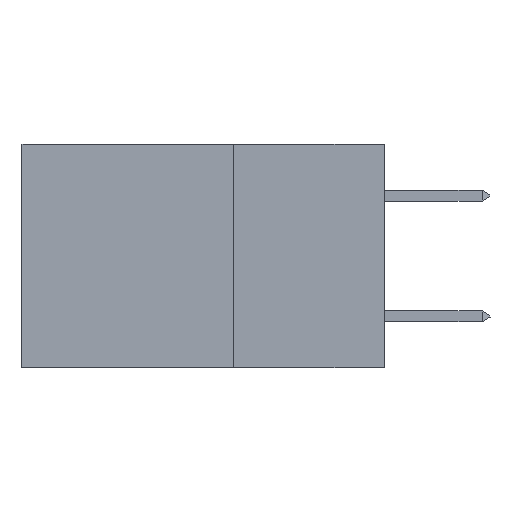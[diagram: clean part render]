
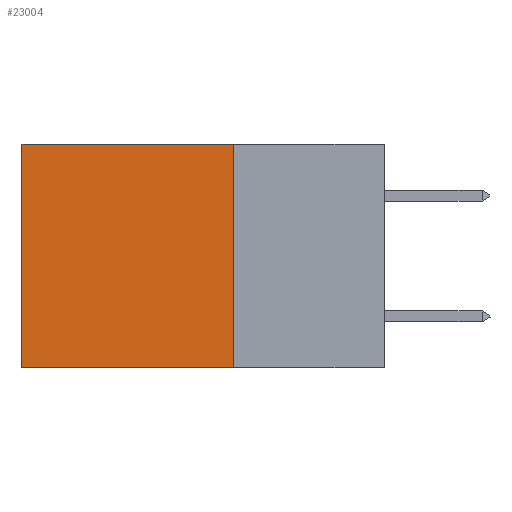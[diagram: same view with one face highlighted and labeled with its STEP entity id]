
A CAD part, left-side view. The second image highlights one B-rep face of the part: STEP entity #23004.
In plain terms, the highlighted planar face has unit normal (-1, 0, 0).
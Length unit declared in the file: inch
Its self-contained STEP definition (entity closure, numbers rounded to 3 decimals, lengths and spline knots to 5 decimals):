
#65 = EDGE_CURVE ( 'NONE', #19885, #15880, #6908, .T. ) ;
#614 = EDGE_CURVE ( 'NONE', #10385, #22251, #22687, .T. ) ;
#1205 = ORIENTED_EDGE ( 'NONE', *, *, #20233, .F. ) ;
#1429 = DIRECTION ( 'NONE',  ( 1., 0., 0. ) ) ;
#2388 = CARTESIAN_POINT ( 'NONE',  ( 0.2875, 0.25, 0. ) ) ;
#2596 = CARTESIAN_POINT ( 'NONE',  ( 0.2875, 0.25, 0. ) ) ;
#2644 = LINE ( 'NONE', #16256, #2942 ) ;
#2942 = VECTOR ( 'NONE', #5748, 39.37008 ) ;
#3942 = CARTESIAN_POINT ( 'NONE',  ( 0.2875, 0.25, -0.37 ) ) ;
#4530 = CARTESIAN_POINT ( 'NONE',  ( 0.2875, 0.6, 0. ) ) ;
#4568 = CARTESIAN_POINT ( 'NONE',  ( 0.2875, 0.6, -0.37 ) ) ;
#5175 = PLANE ( 'NONE',  #17628 ) ;
#5748 = DIRECTION ( 'NONE',  ( 0., 0., -1. ) ) ;
#6045 = ORIENTED_EDGE ( 'NONE', *, *, #614, .F. ) ;
#6600 = VECTOR ( 'NONE', #21650, 39.37008 ) ;
#6729 = ORIENTED_EDGE ( 'NONE', *, *, #8771, .T. ) ;
#6908 = LINE ( 'NONE', #2388, #9150 ) ;
#8771 = EDGE_CURVE ( 'NONE', #15880, #22251, #9084, .T. ) ;
#8780 = DIRECTION ( 'NONE',  ( 0., 0., -1. ) ) ;
#9084 = LINE ( 'NONE', #4530, #19237 ) ;
#9150 = VECTOR ( 'NONE', #18336, 39.37008 ) ;
#9352 = ORIENTED_EDGE ( 'NONE', *, *, #65, .T. ) ;
#10385 = VERTEX_POINT ( 'NONE', #17531 ) ;
#14507 = CARTESIAN_POINT ( 'NONE',  ( 0.2875, 0.6, 0. ) ) ;
#15880 = VERTEX_POINT ( 'NONE', #14507 ) ;
#16256 = CARTESIAN_POINT ( 'NONE',  ( 0.2875, 0.25, 0. ) ) ;
#17531 = CARTESIAN_POINT ( 'NONE',  ( 0.2875, 0.25, -0.37 ) ) ;
#17628 = AXIS2_PLACEMENT_3D ( 'NONE', #19654, #1429, #8780 ) ;
#18336 = DIRECTION ( 'NONE',  ( 0., 1., 0. ) ) ;
#18894 = EDGE_LOOP ( 'NONE', ( #6729, #6045, #1205, #9352 ) ) ;
#19237 = VECTOR ( 'NONE', #20788, 39.37008 ) ;
#19654 = CARTESIAN_POINT ( 'NONE',  ( 0.2875, 0.25, 0. ) ) ;
#19885 = VERTEX_POINT ( 'NONE', #2596 ) ;
#20233 = EDGE_CURVE ( 'NONE', #19885, #10385, #2644, .T. ) ;
#20581 = FACE_OUTER_BOUND ( 'NONE', #18894, .T. ) ;
#20788 = DIRECTION ( 'NONE',  ( 0., 0., -1. ) ) ;
#21650 = DIRECTION ( 'NONE',  ( 0., 1., 0. ) ) ;
#22251 = VERTEX_POINT ( 'NONE', #4568 ) ;
#22687 = LINE ( 'NONE', #3942, #6600 ) ;
#23004 = ADVANCED_FACE ( 'NONE', ( #20581 ), #5175, .F. ) ;
